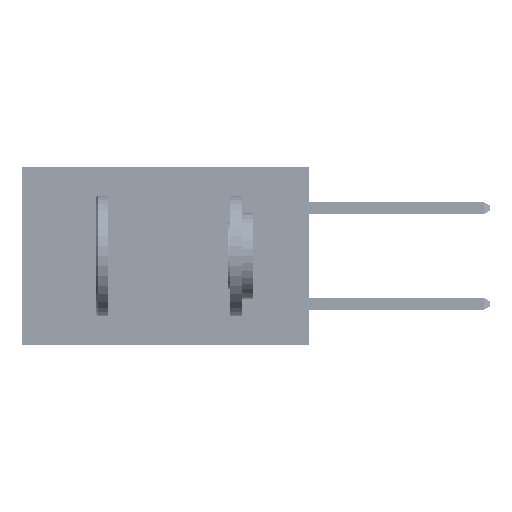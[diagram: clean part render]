
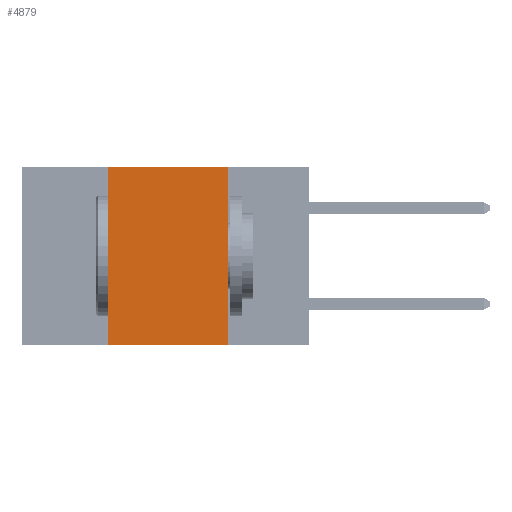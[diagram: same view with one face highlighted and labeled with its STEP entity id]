
A CAD part, left-side view. The second image highlights one B-rep face of the part: STEP entity #4879.
In plain terms, the highlighted planar face has unit normal (-1, 0, 0).
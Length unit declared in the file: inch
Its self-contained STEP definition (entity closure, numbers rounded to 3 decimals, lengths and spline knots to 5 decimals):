
#1285 = VERTEX_POINT ( 'NONE', #7602 ) ;
#2542 = VERTEX_POINT ( 'NONE', #46929 ) ;
#4879 = ADVANCED_FACE ( 'NONE', ( #20773 ), #20875, .F. ) ;
#6500 = EDGE_CURVE ( 'NONE', #36453, #29895, #47348, .T. ) ;
#7602 = CARTESIAN_POINT ( 'NONE',  ( 0., 0.17, 0. ) ) ;
#7825 = VECTOR ( 'NONE', #30394, 39.37008 ) ;
#8265 = CARTESIAN_POINT ( 'NONE',  ( 0., 0.42, 0. ) ) ;
#8418 = ORIENTED_EDGE ( 'NONE', *, *, #41698, .F. ) ;
#12182 = EDGE_CURVE ( 'NONE', #36453, #2542, #23904, .T. ) ;
#13128 = CARTESIAN_POINT ( 'NONE',  ( 0., 0.6, 0. ) ) ;
#13607 = DIRECTION ( 'NONE',  ( 0., 0., -1. ) ) ;
#14272 = EDGE_LOOP ( 'NONE', ( #8418, #26905, #27002, #15776 ) ) ;
#15776 = ORIENTED_EDGE ( 'NONE', *, *, #6500, .T. ) ;
#18913 = CARTESIAN_POINT ( 'NONE',  ( 0., 0.17, -0.37 ) ) ;
#20773 = FACE_OUTER_BOUND ( 'NONE', #14272, .T. ) ;
#20875 = PLANE ( 'NONE',  #39002 ) ;
#23904 = LINE ( 'NONE', #8265, #37803 ) ;
#26905 = ORIENTED_EDGE ( 'NONE', *, *, #27342, .F. ) ;
#26957 = VECTOR ( 'NONE', #37232, 39.37008 ) ;
#27002 = ORIENTED_EDGE ( 'NONE', *, *, #12182, .F. ) ;
#27342 = EDGE_CURVE ( 'NONE', #2542, #1285, #28144, .T. ) ;
#28144 = LINE ( 'NONE', #44382, #26957 ) ;
#28607 = LINE ( 'NONE', #38043, #39663 ) ;
#29895 = VERTEX_POINT ( 'NONE', #18913 ) ;
#30394 = DIRECTION ( 'NONE',  ( 0., -1., 0. ) ) ;
#35826 = DIRECTION ( 'NONE',  ( 1., 0., 0. ) ) ;
#36453 = VERTEX_POINT ( 'NONE', #37928 ) ;
#37232 = DIRECTION ( 'NONE',  ( 0., -1., 0. ) ) ;
#37716 = DIRECTION ( 'NONE',  ( 0., 0., -1. ) ) ;
#37803 = VECTOR ( 'NONE', #38274, 39.37008 ) ;
#37928 = CARTESIAN_POINT ( 'NONE',  ( 0., 0.42, -0.37 ) ) ;
#38043 = CARTESIAN_POINT ( 'NONE',  ( 0., 0.17, 0. ) ) ;
#38274 = DIRECTION ( 'NONE',  ( 0., 0., 1. ) ) ;
#39002 = AXIS2_PLACEMENT_3D ( 'NONE', #13128, #35826, #13607 ) ;
#39663 = VECTOR ( 'NONE', #37716, 39.37008 ) ;
#41698 = EDGE_CURVE ( 'NONE', #1285, #29895, #28607, .T. ) ;
#44382 = CARTESIAN_POINT ( 'NONE',  ( 0., 0.6, 0. ) ) ;
#45157 = CARTESIAN_POINT ( 'NONE',  ( 0., 0.6, -0.37 ) ) ;
#46929 = CARTESIAN_POINT ( 'NONE',  ( 0., 0.42, 0. ) ) ;
#47348 = LINE ( 'NONE', #45157, #7825 ) ;
